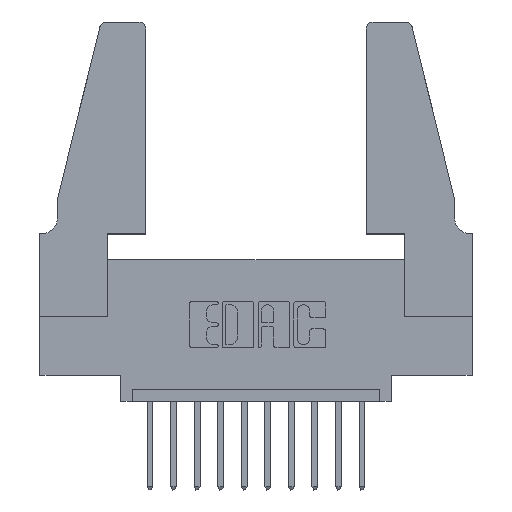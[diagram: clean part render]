
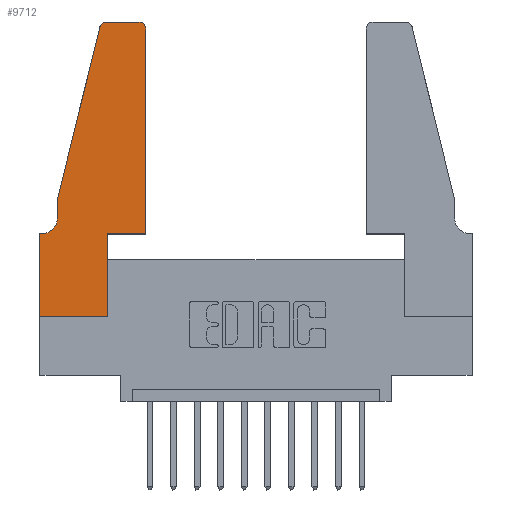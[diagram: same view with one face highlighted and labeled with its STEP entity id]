
A CAD part, top view. The second image highlights one B-rep face of the part: STEP entity #9712.
In plain terms, the highlighted planar face has unit normal (0, 0, 1).
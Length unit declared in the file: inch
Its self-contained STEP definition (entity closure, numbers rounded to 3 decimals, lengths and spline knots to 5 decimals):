
#71 = CIRCLE ( 'NONE', #11274, 0.03 ) ;
#84 = EDGE_CURVE ( 'NONE', #1150, #7387, #9756, .T. ) ;
#225 = DIRECTION ( 'NONE',  ( 1., 0., 0. ) ) ;
#285 = ORIENTED_EDGE ( 'NONE', *, *, #84, .T. ) ;
#339 = CARTESIAN_POINT ( 'NONE',  ( 0.4505, 0.35, 0.37 ) ) ;
#361 = DIRECTION ( 'NONE',  ( 0., 0., -1. ) ) ;
#378 = ORIENTED_EDGE ( 'NONE', *, *, #6947, .T. ) ;
#498 = CARTESIAN_POINT ( 'NONE',  ( 0.0055, 0.42, 0.37 ) ) ;
#572 = EDGE_CURVE ( 'NONE', #12441, #1150, #3622, .T. ) ;
#877 = DIRECTION ( 'NONE',  ( 1., 0., 0. ) ) ;
#921 = CARTESIAN_POINT ( 'NONE',  ( 0.2865, 0.35, 0.37 ) ) ;
#1016 = DIRECTION ( 'NONE',  ( -1., 0., 0. ) ) ;
#1150 = VERTEX_POINT ( 'NONE', #6177 ) ;
#1181 = VECTOR ( 'NONE', #1875, 39.37008 ) ;
#1596 = LINE ( 'NONE', #9050, #12881 ) ;
#1637 = CARTESIAN_POINT ( 'NONE',  ( 0.0755, 0.5, 0.37 ) ) ;
#1779 = ORIENTED_EDGE ( 'NONE', *, *, #13952, .T. ) ;
#1786 = VECTOR ( 'NONE', #11169, 39.37008 ) ;
#1819 = CARTESIAN_POINT ( 'NONE',  ( 0.0055, 0.35, 0.37 ) ) ;
#1875 = DIRECTION ( 'NONE',  ( 0., 1., 0. ) ) ;
#1881 = VERTEX_POINT ( 'NONE', #13183 ) ;
#2117 = EDGE_CURVE ( 'NONE', #11203, #6938, #4112, .T. ) ;
#2226 = EDGE_CURVE ( 'NONE', #14051, #7349, #10601, .T. ) ;
#2577 = VERTEX_POINT ( 'NONE', #5202 ) ;
#3118 = PLANE ( 'NONE',  #3461 ) ;
#3277 = AXIS2_PLACEMENT_3D ( 'NONE', #7763, #13131, #225 ) ;
#3310 = ORIENTED_EDGE ( 'NONE', *, *, #2117, .T. ) ;
#3325 = LINE ( 'NONE', #7606, #8837 ) ;
#3373 = VECTOR ( 'NONE', #9303, 39.37008 ) ;
#3461 = AXIS2_PLACEMENT_3D ( 'NONE', #9512, #11879, #877 ) ;
#3607 = FACE_OUTER_BOUND ( 'NONE', #11860, .T. ) ;
#3622 = LINE ( 'NONE', #6913, #6225 ) ;
#3811 = ORIENTED_EDGE ( 'NONE', *, *, #10358, .T. ) ;
#4112 = CIRCLE ( 'NONE', #6096, 0.07 ) ;
#4215 = DIRECTION ( 'NONE',  ( -0.239, -0.971, 0. ) ) ;
#4555 = ORIENTED_EDGE ( 'NONE', *, *, #5746, .T. ) ;
#4601 = CARTESIAN_POINT ( 'NONE',  ( 0.0755, 0.5, 0.37 ) ) ;
#5173 = LINE ( 'NONE', #8475, #8072 ) ;
#5202 = CARTESIAN_POINT ( 'NONE',  ( 0.4505, 1.22, 0.37 ) ) ;
#5205 = CARTESIAN_POINT ( 'NONE',  ( 0., 0., 0.37 ) ) ;
#5250 = LINE ( 'NONE', #5205, #12247 ) ;
#5746 = EDGE_CURVE ( 'NONE', #6938, #1881, #3325, .T. ) ;
#5974 = VERTEX_POINT ( 'NONE', #11718 ) ;
#6007 = DIRECTION ( 'NONE',  ( 1., 0., 0. ) ) ;
#6096 = AXIS2_PLACEMENT_3D ( 'NONE', #498, #361, #8033 ) ;
#6177 = CARTESIAN_POINT ( 'NONE',  ( 0.284, 1.25, 0.37 ) ) ;
#6225 = VECTOR ( 'NONE', #13288, 39.37008 ) ;
#6397 = EDGE_CURVE ( 'NONE', #5974, #2577, #10364, .T. ) ;
#6628 = VERTEX_POINT ( 'NONE', #9982 ) ;
#6707 = CARTESIAN_POINT ( 'NONE',  ( 0.4505, 0.35, 0.37 ) ) ;
#6913 = CARTESIAN_POINT ( 'NONE',  ( 0.2605, 1.25, 0.37 ) ) ;
#6938 = VERTEX_POINT ( 'NONE', #1819 ) ;
#6947 = EDGE_CURVE ( 'NONE', #1881, #6628, #5250, .T. ) ;
#7349 = VERTEX_POINT ( 'NONE', #8063 ) ;
#7359 = LINE ( 'NONE', #1637, #3373 ) ;
#7387 = VERTEX_POINT ( 'NONE', #9068 ) ;
#7492 = ORIENTED_EDGE ( 'NONE', *, *, #8864, .T. ) ;
#7606 = CARTESIAN_POINT ( 'NONE',  ( 0.0755, 0.35, 0.37 ) ) ;
#7763 = CARTESIAN_POINT ( 'NONE',  ( 0.284, 1.22, 0.37 ) ) ;
#8033 = DIRECTION ( 'NONE',  ( -1., 0., 0. ) ) ;
#8063 = CARTESIAN_POINT ( 'NONE',  ( 0.2865, 0.35, 0.37 ) ) ;
#8072 = VECTOR ( 'NONE', #4215, 39.37008 ) ;
#8475 = CARTESIAN_POINT ( 'NONE',  ( 0.0755, 0.5, 0.37 ) ) ;
#8576 = ORIENTED_EDGE ( 'NONE', *, *, #13204, .T. ) ;
#8837 = VECTOR ( 'NONE', #1016, 39.37008 ) ;
#8864 = EDGE_CURVE ( 'NONE', #6628, #14051, #1596, .T. ) ;
#9050 = CARTESIAN_POINT ( 'NONE',  ( 0., 0., 0.37 ) ) ;
#9068 = CARTESIAN_POINT ( 'NONE',  ( 0.25487, 1.22718, 0.37 ) ) ;
#9303 = DIRECTION ( 'NONE',  ( 0., -1., 0. ) ) ;
#9366 = CARTESIAN_POINT ( 'NONE',  ( 0.4205, 1.22, 0.37 ) ) ;
#9512 = CARTESIAN_POINT ( 'NONE',  ( 0., 0.35, 0.37 ) ) ;
#9712 = ADVANCED_FACE ( 'NONE', ( #3607 ), #3118, .T. ) ;
#9756 = CIRCLE ( 'NONE', #3277, 0.03 ) ;
#9910 = ORIENTED_EDGE ( 'NONE', *, *, #2226, .T. ) ;
#9960 = ORIENTED_EDGE ( 'NONE', *, *, #6397, .T. ) ;
#9965 = CARTESIAN_POINT ( 'NONE',  ( 0.4205, 1.25, 0.37 ) ) ;
#9982 = CARTESIAN_POINT ( 'NONE',  ( 0., 0., 0.37 ) ) ;
#10153 = DIRECTION ( 'NONE',  ( 1., 0., 0. ) ) ;
#10155 = VECTOR ( 'NONE', #6007, 39.37008 ) ;
#10358 = EDGE_CURVE ( 'NONE', #7387, #11940, #5173, .T. ) ;
#10364 = LINE ( 'NONE', #6707, #1786 ) ;
#10416 = ORIENTED_EDGE ( 'NONE', *, *, #12043, .T. ) ;
#10601 = LINE ( 'NONE', #921, #1181 ) ;
#11054 = ORIENTED_EDGE ( 'NONE', *, *, #572, .T. ) ;
#11169 = DIRECTION ( 'NONE',  ( 0., 1., 0. ) ) ;
#11203 = VERTEX_POINT ( 'NONE', #11210 ) ;
#11210 = CARTESIAN_POINT ( 'NONE',  ( 0.0755, 0.42, 0.37 ) ) ;
#11274 = AXIS2_PLACEMENT_3D ( 'NONE', #9366, #12555, #13734 ) ;
#11718 = CARTESIAN_POINT ( 'NONE',  ( 0.4505, 0.35, 0.37 ) ) ;
#11860 = EDGE_LOOP ( 'NONE', ( #11054, #285, #3811, #10416, #3310, #4555, #378, #7492, #9910, #1779, #9960, #8576 ) ) ;
#11879 = DIRECTION ( 'NONE',  ( 0., 0., 1. ) ) ;
#11940 = VERTEX_POINT ( 'NONE', #4601 ) ;
#12043 = EDGE_CURVE ( 'NONE', #11940, #11203, #7359, .T. ) ;
#12247 = VECTOR ( 'NONE', #12826, 39.37008 ) ;
#12357 = LINE ( 'NONE', #339, #10155 ) ;
#12441 = VERTEX_POINT ( 'NONE', #9965 ) ;
#12555 = DIRECTION ( 'NONE',  ( 0., 0., 1. ) ) ;
#12826 = DIRECTION ( 'NONE',  ( 0., -1., 0. ) ) ;
#12881 = VECTOR ( 'NONE', #10153, 39.37008 ) ;
#13131 = DIRECTION ( 'NONE',  ( 0., 0., 1. ) ) ;
#13183 = CARTESIAN_POINT ( 'NONE',  ( 0., 0.35, 0.37 ) ) ;
#13204 = EDGE_CURVE ( 'NONE', #2577, #12441, #71, .T. ) ;
#13288 = DIRECTION ( 'NONE',  ( -1., 0., 0. ) ) ;
#13669 = CARTESIAN_POINT ( 'NONE',  ( 0.2865, 0., 0.37 ) ) ;
#13734 = DIRECTION ( 'NONE',  ( 1., 0., 0. ) ) ;
#13952 = EDGE_CURVE ( 'NONE', #7349, #5974, #12357, .T. ) ;
#14051 = VERTEX_POINT ( 'NONE', #13669 ) ;
